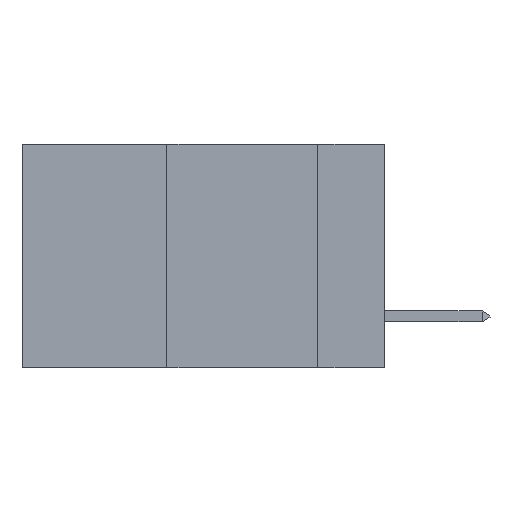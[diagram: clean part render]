
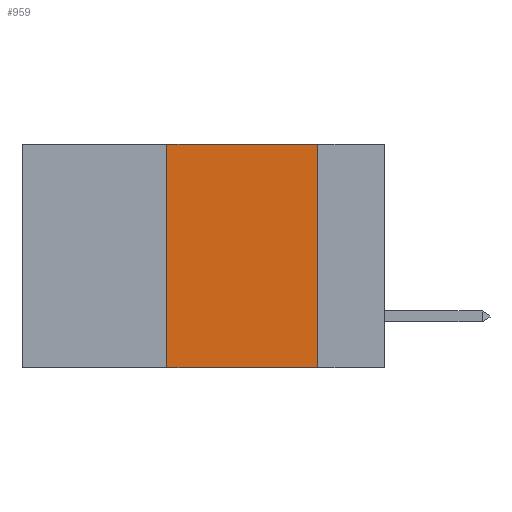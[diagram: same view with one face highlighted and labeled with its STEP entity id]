
A CAD part, left-side view. The second image highlights one B-rep face of the part: STEP entity #959.
In plain terms, the highlighted planar face has unit normal (-1, 0, 0).
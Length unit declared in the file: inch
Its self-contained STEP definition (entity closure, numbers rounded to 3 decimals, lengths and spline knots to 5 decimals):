
#60 = AXIS2_PLACEMENT_3D ( 'NONE', #8686, #2381, #14141 ) ;
#248 = VERTEX_POINT ( 'NONE', #974 ) ;
#712 = VERTEX_POINT ( 'NONE', #2335 ) ;
#959 = ADVANCED_FACE ( 'NONE', ( #7329 ), #3450, .F. ) ;
#974 = CARTESIAN_POINT ( 'NONE',  ( 0., 0.36, 0. ) ) ;
#1278 = VERTEX_POINT ( 'NONE', #13009 ) ;
#1803 = CARTESIAN_POINT ( 'NONE',  ( 0., 0.36, -0.37 ) ) ;
#2335 = CARTESIAN_POINT ( 'NONE',  ( 0., 0.11, 0. ) ) ;
#2381 = DIRECTION ( 'NONE',  ( 1., 0., 0. ) ) ;
#2596 = LINE ( 'NONE', #6032, #6470 ) ;
#3415 = ORIENTED_EDGE ( 'NONE', *, *, #8018, .F. ) ;
#3450 = PLANE ( 'NONE',  #60 ) ;
#3553 = VECTOR ( 'NONE', #16938, 39.37008 ) ;
#4010 = EDGE_LOOP ( 'NONE', ( #6341, #13381, #3415, #10426 ) ) ;
#4335 = VERTEX_POINT ( 'NONE', #1803 ) ;
#4835 = EDGE_CURVE ( 'NONE', #248, #712, #12903, .T. ) ;
#5215 = LINE ( 'NONE', #12448, #11543 ) ;
#6032 = CARTESIAN_POINT ( 'NONE',  ( 0., 0.36, 0. ) ) ;
#6341 = ORIENTED_EDGE ( 'NONE', *, *, #7975, .F. ) ;
#6470 = VECTOR ( 'NONE', #14737, 39.37008 ) ;
#7204 = CARTESIAN_POINT ( 'NONE',  ( 0., 0.11, 0. ) ) ;
#7329 = FACE_OUTER_BOUND ( 'NONE', #4010, .T. ) ;
#7911 = DIRECTION ( 'NONE',  ( 0., -1., 0. ) ) ;
#7975 = EDGE_CURVE ( 'NONE', #712, #1278, #13874, .T. ) ;
#8018 = EDGE_CURVE ( 'NONE', #4335, #248, #2596, .T. ) ;
#8095 = EDGE_CURVE ( 'NONE', #4335, #1278, #5215, .T. ) ;
#8686 = CARTESIAN_POINT ( 'NONE',  ( 0., 0.6, 0. ) ) ;
#10426 = ORIENTED_EDGE ( 'NONE', *, *, #8095, .T. ) ;
#11543 = VECTOR ( 'NONE', #13698, 39.37008 ) ;
#11574 = CARTESIAN_POINT ( 'NONE',  ( 0., 0.6, 0. ) ) ;
#12448 = CARTESIAN_POINT ( 'NONE',  ( 0., 0.6, -0.37 ) ) ;
#12903 = LINE ( 'NONE', #11574, #15729 ) ;
#13009 = CARTESIAN_POINT ( 'NONE',  ( 0., 0.11, -0.37 ) ) ;
#13381 = ORIENTED_EDGE ( 'NONE', *, *, #4835, .F. ) ;
#13698 = DIRECTION ( 'NONE',  ( 0., -1., 0. ) ) ;
#13874 = LINE ( 'NONE', #7204, #3553 ) ;
#14141 = DIRECTION ( 'NONE',  ( 0., 0., -1. ) ) ;
#14737 = DIRECTION ( 'NONE',  ( 0., 0., 1. ) ) ;
#15729 = VECTOR ( 'NONE', #7911, 39.37008 ) ;
#16938 = DIRECTION ( 'NONE',  ( 0., 0., -1. ) ) ;
